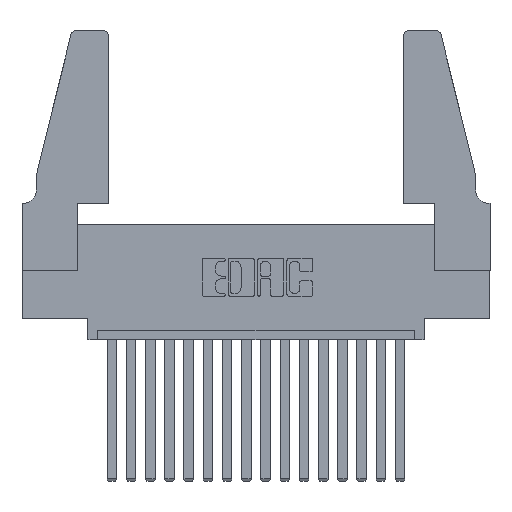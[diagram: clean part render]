
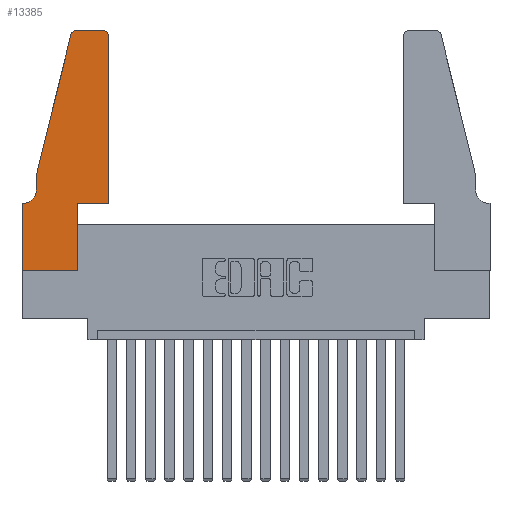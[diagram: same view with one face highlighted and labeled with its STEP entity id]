
A CAD part, top view. The second image highlights one B-rep face of the part: STEP entity #13385.
In plain terms, the highlighted planar face has unit normal (0, 0, 1).
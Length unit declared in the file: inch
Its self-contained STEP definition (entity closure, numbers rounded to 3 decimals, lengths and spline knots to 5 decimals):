
#73 = LINE ( 'NONE', #13190, #15010 ) ;
#186 = VERTEX_POINT ( 'NONE', #11043 ) ;
#728 = EDGE_CURVE ( 'NONE', #4155, #11036, #16981, .T. ) ;
#1067 = EDGE_CURVE ( 'NONE', #13667, #4500, #7386, .T. ) ;
#1450 = EDGE_CURVE ( 'NONE', #8098, #3572, #1605, .T. ) ;
#1501 = EDGE_CURVE ( 'NONE', #12758, #4155, #12673, .T. ) ;
#1605 = LINE ( 'NONE', #14080, #15248 ) ;
#1801 = CARTESIAN_POINT ( 'NONE',  ( 0., 0., 0.37 ) ) ;
#1804 = CARTESIAN_POINT ( 'NONE',  ( 0.0755, 0.42, 0.37 ) ) ;
#1982 = PLANE ( 'NONE',  #7280 ) ;
#2160 = VECTOR ( 'NONE', #3505, 39.37008 ) ;
#2204 = CARTESIAN_POINT ( 'NONE',  ( 0.284, 1.22, 0.37 ) ) ;
#3009 = DIRECTION ( 'NONE',  ( 0., 0., 1. ) ) ;
#3068 = EDGE_CURVE ( 'NONE', #6239, #186, #8998, .T. ) ;
#3236 = CARTESIAN_POINT ( 'NONE',  ( 0.0755, 0.5, 0.37 ) ) ;
#3350 = CARTESIAN_POINT ( 'NONE',  ( 0.0755, 0.35, 0.37 ) ) ;
#3505 = DIRECTION ( 'NONE',  ( 0., 1., 0. ) ) ;
#3514 = VERTEX_POINT ( 'NONE', #8172 ) ;
#3572 = VERTEX_POINT ( 'NONE', #13836 ) ;
#3976 = DIRECTION ( 'NONE',  ( 0., 0., 1. ) ) ;
#4001 = CARTESIAN_POINT ( 'NONE',  ( 0.0755, 0.5, 0.37 ) ) ;
#4135 = ORIENTED_EDGE ( 'NONE', *, *, #10751, .T. ) ;
#4155 = VERTEX_POINT ( 'NONE', #7317 ) ;
#4160 = CARTESIAN_POINT ( 'NONE',  ( 0.2605, 1.25, 0.37 ) ) ;
#4500 = VERTEX_POINT ( 'NONE', #4001 ) ;
#4528 = DIRECTION ( 'NONE',  ( 0., 0., 1. ) ) ;
#4599 = DIRECTION ( 'NONE',  ( -0.239, -0.971, 0. ) ) ;
#4989 = EDGE_CURVE ( 'NONE', #3514, #6239, #7425, .T. ) ;
#5088 = LINE ( 'NONE', #13615, #11889 ) ;
#5420 = ORIENTED_EDGE ( 'NONE', *, *, #10344, .T. ) ;
#5742 = DIRECTION ( 'NONE',  ( 1., 0., 0. ) ) ;
#5768 = LINE ( 'NONE', #6185, #2160 ) ;
#5785 = CARTESIAN_POINT ( 'NONE',  ( 0.0055, 0.35, 0.37 ) ) ;
#5914 = DIRECTION ( 'NONE',  ( 1., 0., 0. ) ) ;
#6136 = ORIENTED_EDGE ( 'NONE', *, *, #11650, .T. ) ;
#6185 = CARTESIAN_POINT ( 'NONE',  ( 0.4505, 0.35, 0.37 ) ) ;
#6239 = VERTEX_POINT ( 'NONE', #15276 ) ;
#6314 = VECTOR ( 'NONE', #17283, 39.37008 ) ;
#6515 = DIRECTION ( 'NONE',  ( 0., 0., -1. ) ) ;
#6821 = CIRCLE ( 'NONE', #7263, 0.03 ) ;
#7117 = CARTESIAN_POINT ( 'NONE',  ( 0.4205, 1.22, 0.37 ) ) ;
#7263 = AXIS2_PLACEMENT_3D ( 'NONE', #2204, #3976, #14936 ) ;
#7280 = AXIS2_PLACEMENT_3D ( 'NONE', #17029, #4528, #11474 ) ;
#7301 = CARTESIAN_POINT ( 'NONE',  ( 0.0055, 0.42, 0.37 ) ) ;
#7317 = CARTESIAN_POINT ( 'NONE',  ( 0., 0.35, 0.37 ) ) ;
#7348 = EDGE_LOOP ( 'NONE', ( #13193, #7561, #9758, #10578, #4135, #14684, #13643, #13098, #6136, #13686, #5420, #15496 ) ) ;
#7386 = LINE ( 'NONE', #3236, #10777 ) ;
#7425 = CIRCLE ( 'NONE', #17343, 0.03 ) ;
#7463 = DIRECTION ( 'NONE',  ( -1., 0., 0. ) ) ;
#7561 = ORIENTED_EDGE ( 'NONE', *, *, #10522, .T. ) ;
#8098 = VERTEX_POINT ( 'NONE', #17332 ) ;
#8172 = CARTESIAN_POINT ( 'NONE',  ( 0.4505, 1.22, 0.37 ) ) ;
#8300 = CARTESIAN_POINT ( 'NONE',  ( 0.25487, 1.22718, 0.37 ) ) ;
#8516 = AXIS2_PLACEMENT_3D ( 'NONE', #7301, #6515, #9307 ) ;
#8550 = CARTESIAN_POINT ( 'NONE',  ( 0.2865, 0., 0.37 ) ) ;
#8998 = LINE ( 'NONE', #4160, #9415 ) ;
#9307 = DIRECTION ( 'NONE',  ( -1., 0., 0. ) ) ;
#9415 = VECTOR ( 'NONE', #15249, 39.37008 ) ;
#9758 = ORIENTED_EDGE ( 'NONE', *, *, #1067, .T. ) ;
#10041 = VERTEX_POINT ( 'NONE', #1804 ) ;
#10344 = EDGE_CURVE ( 'NONE', #3572, #3514, #5768, .T. ) ;
#10522 = EDGE_CURVE ( 'NONE', #186, #13667, #6821, .T. ) ;
#10578 = ORIENTED_EDGE ( 'NONE', *, *, #14388, .T. ) ;
#10646 = VERTEX_POINT ( 'NONE', #8550 ) ;
#10751 = EDGE_CURVE ( 'NONE', #10041, #12758, #12363, .T. ) ;
#10777 = VECTOR ( 'NONE', #4599, 39.37008 ) ;
#11036 = VERTEX_POINT ( 'NONE', #12627 ) ;
#11043 = CARTESIAN_POINT ( 'NONE',  ( 0.284, 1.25, 0.37 ) ) ;
#11474 = DIRECTION ( 'NONE',  ( 1., 0., 0. ) ) ;
#11650 = EDGE_CURVE ( 'NONE', #10646, #8098, #5088, .T. ) ;
#11889 = VECTOR ( 'NONE', #12296, 39.37008 ) ;
#12245 = VECTOR ( 'NONE', #7463, 39.37008 ) ;
#12262 = FACE_OUTER_BOUND ( 'NONE', #7348, .T. ) ;
#12296 = DIRECTION ( 'NONE',  ( 0., 1., 0. ) ) ;
#12363 = CIRCLE ( 'NONE', #8516, 0.07 ) ;
#12627 = CARTESIAN_POINT ( 'NONE',  ( 0., 0., 0.37 ) ) ;
#12673 = LINE ( 'NONE', #3350, #12245 ) ;
#12758 = VERTEX_POINT ( 'NONE', #5785 ) ;
#13098 = ORIENTED_EDGE ( 'NONE', *, *, #16026, .T. ) ;
#13190 = CARTESIAN_POINT ( 'NONE',  ( 0.0755, 0.5, 0.37 ) ) ;
#13193 = ORIENTED_EDGE ( 'NONE', *, *, #3068, .T. ) ;
#13385 = ADVANCED_FACE ( 'NONE', ( #12262 ), #1982, .T. ) ;
#13615 = CARTESIAN_POINT ( 'NONE',  ( 0.2865, 0.35, 0.37 ) ) ;
#13643 = ORIENTED_EDGE ( 'NONE', *, *, #728, .T. ) ;
#13667 = VERTEX_POINT ( 'NONE', #8300 ) ;
#13686 = ORIENTED_EDGE ( 'NONE', *, *, #1450, .T. ) ;
#13836 = CARTESIAN_POINT ( 'NONE',  ( 0.4505, 0.35, 0.37 ) ) ;
#14080 = CARTESIAN_POINT ( 'NONE',  ( 0.4505, 0.35, 0.37 ) ) ;
#14388 = EDGE_CURVE ( 'NONE', #4500, #10041, #73, .T. ) ;
#14679 = CARTESIAN_POINT ( 'NONE',  ( 0., 0., 0.37 ) ) ;
#14684 = ORIENTED_EDGE ( 'NONE', *, *, #1501, .T. ) ;
#14936 = DIRECTION ( 'NONE',  ( 1., 0., 0. ) ) ;
#15010 = VECTOR ( 'NONE', #17180, 39.37008 ) ;
#15248 = VECTOR ( 'NONE', #5914, 39.37008 ) ;
#15249 = DIRECTION ( 'NONE',  ( -1., 0., 0. ) ) ;
#15276 = CARTESIAN_POINT ( 'NONE',  ( 0.4205, 1.25, 0.37 ) ) ;
#15496 = ORIENTED_EDGE ( 'NONE', *, *, #4989, .T. ) ;
#16026 = EDGE_CURVE ( 'NONE', #11036, #10646, #16812, .T. ) ;
#16812 = LINE ( 'NONE', #1801, #17206 ) ;
#16920 = DIRECTION ( 'NONE',  ( 1., 0., 0. ) ) ;
#16981 = LINE ( 'NONE', #14679, #6314 ) ;
#17029 = CARTESIAN_POINT ( 'NONE',  ( 0., 0.35, 0.37 ) ) ;
#17180 = DIRECTION ( 'NONE',  ( 0., -1., 0. ) ) ;
#17206 = VECTOR ( 'NONE', #16920, 39.37008 ) ;
#17283 = DIRECTION ( 'NONE',  ( 0., -1., 0. ) ) ;
#17332 = CARTESIAN_POINT ( 'NONE',  ( 0.2865, 0.35, 0.37 ) ) ;
#17343 = AXIS2_PLACEMENT_3D ( 'NONE', #7117, #3009, #5742 ) ;
